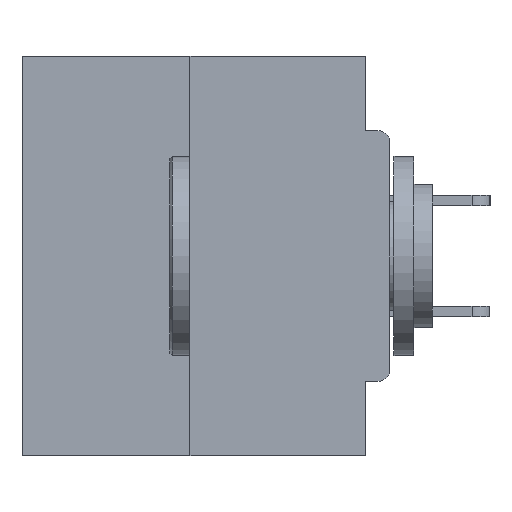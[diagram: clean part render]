
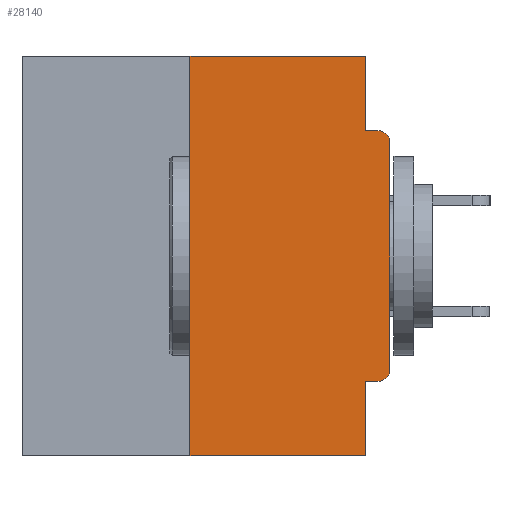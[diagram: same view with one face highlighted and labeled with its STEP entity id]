
A CAD part, left-side view. The second image highlights one B-rep face of the part: STEP entity #28140.
In plain terms, the highlighted planar face has unit normal (-1, 0, 0).
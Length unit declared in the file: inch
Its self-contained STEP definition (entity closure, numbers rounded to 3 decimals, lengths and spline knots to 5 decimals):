
#137 = ORIENTED_EDGE ( 'NONE', *, *, #13749, .F. ) ;
#266 = DIRECTION ( 'NONE',  ( 0., 0., -1. ) ) ;
#646 = VECTOR ( 'NONE', #4612, 39.37008 ) ;
#818 = VERTEX_POINT ( 'NONE', #7182 ) ;
#1011 = EDGE_CURVE ( 'NONE', #22884, #33250, #3286, .T. ) ;
#1149 = VERTEX_POINT ( 'NONE', #27152 ) ;
#2269 = VECTOR ( 'NONE', #31890, 39.37008 ) ;
#2272 = DIRECTION ( 'NONE',  ( -1., 0., 0. ) ) ;
#2774 = DIRECTION ( 'NONE',  ( 0., 0., -1. ) ) ;
#3286 = LINE ( 'NONE', #5010, #7808 ) ;
#4051 = VECTOR ( 'NONE', #4407, 39.37008 ) ;
#4344 = DIRECTION ( 'NONE',  ( 0., -1., 0. ) ) ;
#4407 = DIRECTION ( 'NONE',  ( 0., 0., 1. ) ) ;
#4596 = CIRCLE ( 'NONE', #17506, 0.015 ) ;
#4612 = DIRECTION ( 'NONE',  ( 0., 0., 1. ) ) ;
#5010 = CARTESIAN_POINT ( 'NONE',  ( 0., 0.46, 0. ) ) ;
#5126 = CARTESIAN_POINT ( 'NONE',  ( 0., 0.015, -0.4065 ) ) ;
#5230 = DIRECTION ( 'NONE',  ( 0., -1., 0. ) ) ;
#5387 = LINE ( 'NONE', #25701, #6605 ) ;
#5653 = CARTESIAN_POINT ( 'NONE',  ( 0., 0.015, -0.1085 ) ) ;
#6605 = VECTOR ( 'NONE', #17957, 39.37008 ) ;
#6793 = ORIENTED_EDGE ( 'NONE', *, *, #28416, .F. ) ;
#7182 = CARTESIAN_POINT ( 'NONE',  ( 0., 0.031, -0.5 ) ) ;
#7256 = AXIS2_PLACEMENT_3D ( 'NONE', #25106, #30756, #27993 ) ;
#7808 = VECTOR ( 'NONE', #5230, 39.37008 ) ;
#8527 = EDGE_CURVE ( 'NONE', #8582, #27568, #4596, .T. ) ;
#8540 = CARTESIAN_POINT ( 'NONE',  ( 0., 0., -0.1085 ) ) ;
#8582 = VERTEX_POINT ( 'NONE', #5126 ) ;
#8627 = DIRECTION ( 'NONE',  ( -1., 0., 0. ) ) ;
#9330 = ORIENTED_EDGE ( 'NONE', *, *, #18900, .F. ) ;
#9836 = PLANE ( 'NONE',  #7256 ) ;
#10490 = ORIENTED_EDGE ( 'NONE', *, *, #24950, .T. ) ;
#10617 = VERTEX_POINT ( 'NONE', #8540 ) ;
#10913 = LINE ( 'NONE', #22865, #646 ) ;
#10994 = CIRCLE ( 'NONE', #33928, 0.015 ) ;
#11675 = CARTESIAN_POINT ( 'NONE',  ( 0., 0.25, -0.5 ) ) ;
#12189 = ORIENTED_EDGE ( 'NONE', *, *, #14023, .T. ) ;
#12727 = ORIENTED_EDGE ( 'NONE', *, *, #1011, .F. ) ;
#13749 = EDGE_CURVE ( 'NONE', #33250, #30755, #16135, .T. ) ;
#14023 = EDGE_CURVE ( 'NONE', #31380, #818, #27310, .T. ) ;
#14927 = VECTOR ( 'NONE', #2774, 39.37008 ) ;
#15156 = LINE ( 'NONE', #15636, #27405 ) ;
#15200 = ORIENTED_EDGE ( 'NONE', *, *, #31269, .T. ) ;
#15499 = CARTESIAN_POINT ( 'NONE',  ( 0., 0.031, 0. ) ) ;
#15636 = CARTESIAN_POINT ( 'NONE',  ( 0., 0., -0.0935 ) ) ;
#15826 = EDGE_LOOP ( 'NONE', ( #12727, #33427, #12189, #9330, #16316, #19691, #15200, #10490, #6793, #137 ) ) ;
#16135 = LINE ( 'NONE', #15499, #14927 ) ;
#16316 = ORIENTED_EDGE ( 'NONE', *, *, #16529, .F. ) ;
#16529 = EDGE_CURVE ( 'NONE', #8582, #26507, #18235, .T. ) ;
#17506 = AXIS2_PLACEMENT_3D ( 'NONE', #28684, #2272, #23379 ) ;
#17957 = DIRECTION ( 'NONE',  ( 0., 0., -1. ) ) ;
#18129 = CARTESIAN_POINT ( 'NONE',  ( 0., 0.25, 0. ) ) ;
#18235 = LINE ( 'NONE', #28993, #2269 ) ;
#18284 = VECTOR ( 'NONE', #4344, 39.37008 ) ;
#18900 = EDGE_CURVE ( 'NONE', #26507, #818, #5387, .T. ) ;
#19691 = ORIENTED_EDGE ( 'NONE', *, *, #8527, .T. ) ;
#22865 = CARTESIAN_POINT ( 'NONE',  ( 0., 0., 0. ) ) ;
#22884 = VERTEX_POINT ( 'NONE', #30010 ) ;
#23379 = DIRECTION ( 'NONE',  ( 0., 0., -1. ) ) ;
#23907 = EDGE_CURVE ( 'NONE', #31380, #22884, #33179, .T. ) ;
#24950 = EDGE_CURVE ( 'NONE', #10617, #1149, #10994, .T. ) ;
#25106 = CARTESIAN_POINT ( 'NONE',  ( 0., 0.46, 0. ) ) ;
#25701 = CARTESIAN_POINT ( 'NONE',  ( 0., 0.031, -0.5 ) ) ;
#25884 = DIRECTION ( 'NONE',  ( 0., -1., 0. ) ) ;
#26507 = VERTEX_POINT ( 'NONE', #27024 ) ;
#26878 = CARTESIAN_POINT ( 'NONE',  ( 0., 0.031, 0. ) ) ;
#27008 = FACE_OUTER_BOUND ( 'NONE', #15826, .T. ) ;
#27024 = CARTESIAN_POINT ( 'NONE',  ( 0., 0.031, -0.4065 ) ) ;
#27152 = CARTESIAN_POINT ( 'NONE',  ( 0., 0.015, -0.0935 ) ) ;
#27310 = LINE ( 'NONE', #30544, #18284 ) ;
#27405 = VECTOR ( 'NONE', #25884, 39.37008 ) ;
#27568 = VERTEX_POINT ( 'NONE', #30679 ) ;
#27993 = DIRECTION ( 'NONE',  ( 0., 0., -1. ) ) ;
#28140 = ADVANCED_FACE ( 'NONE', ( #27008 ), #9836, .F. ) ;
#28416 = EDGE_CURVE ( 'NONE', #30755, #1149, #15156, .T. ) ;
#28684 = CARTESIAN_POINT ( 'NONE',  ( 0., 0.015, -0.3915 ) ) ;
#28774 = CARTESIAN_POINT ( 'NONE',  ( 0., 0.031, -0.0935 ) ) ;
#28993 = CARTESIAN_POINT ( 'NONE',  ( 0., 0., -0.4065 ) ) ;
#30010 = CARTESIAN_POINT ( 'NONE',  ( 0., 0.25, 0. ) ) ;
#30544 = CARTESIAN_POINT ( 'NONE',  ( 0., 0.46, -0.5 ) ) ;
#30679 = CARTESIAN_POINT ( 'NONE',  ( 0., 0., -0.3915 ) ) ;
#30755 = VERTEX_POINT ( 'NONE', #28774 ) ;
#30756 = DIRECTION ( 'NONE',  ( 1., 0., 0. ) ) ;
#31269 = EDGE_CURVE ( 'NONE', #27568, #10617, #10913, .T. ) ;
#31380 = VERTEX_POINT ( 'NONE', #11675 ) ;
#31890 = DIRECTION ( 'NONE',  ( 0., 1., 0. ) ) ;
#33179 = LINE ( 'NONE', #18129, #4051 ) ;
#33250 = VERTEX_POINT ( 'NONE', #26878 ) ;
#33427 = ORIENTED_EDGE ( 'NONE', *, *, #23907, .F. ) ;
#33928 = AXIS2_PLACEMENT_3D ( 'NONE', #5653, #8627, #266 ) ;
